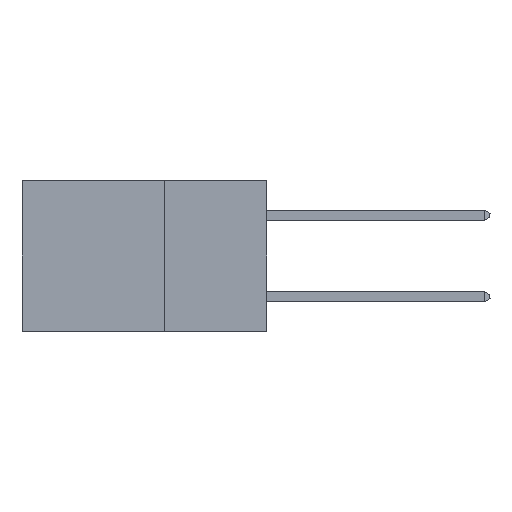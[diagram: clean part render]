
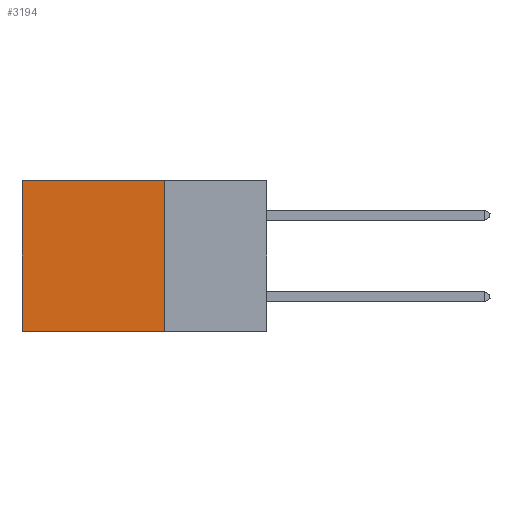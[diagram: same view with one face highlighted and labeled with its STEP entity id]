
A CAD part, left-side view. The second image highlights one B-rep face of the part: STEP entity #3194.
In plain terms, the highlighted planar face has unit normal (-1, 0, 0).
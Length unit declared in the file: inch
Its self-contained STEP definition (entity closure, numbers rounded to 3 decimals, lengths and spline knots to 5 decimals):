
#4 = ORIENTED_EDGE ( 'NONE', *, *, #1946, .F. ) ;
#265 = CARTESIAN_POINT ( 'NONE',  ( 0.2875, 0.6, 0. ) ) ;
#291 = PLANE ( 'NONE',  #7853 ) ;
#560 = CARTESIAN_POINT ( 'NONE',  ( 0.2875, 0.6, -0.37 ) ) ;
#1156 = EDGE_CURVE ( 'NONE', #4462, #20566, #4617, .T. ) ;
#1946 = EDGE_CURVE ( 'NONE', #16893, #4462, #17505, .T. ) ;
#2286 = EDGE_CURVE ( 'NONE', #20542, #20566, #9073, .T. ) ;
#2630 = LINE ( 'NONE', #16672, #20122 ) ;
#2708 = CARTESIAN_POINT ( 'NONE',  ( 0.2875, 0.25, -0.37 ) ) ;
#2721 = CARTESIAN_POINT ( 'NONE',  ( 0.2875, 0.25, 0. ) ) ;
#3194 = ADVANCED_FACE ( 'NONE', ( #3804 ), #291, .F. ) ;
#3804 = FACE_OUTER_BOUND ( 'NONE', #18959, .T. ) ;
#4462 = VERTEX_POINT ( 'NONE', #12052 ) ;
#4510 = DIRECTION ( 'NONE',  ( 0., 1., 0. ) ) ;
#4617 = LINE ( 'NONE', #2708, #19603 ) ;
#5683 = DIRECTION ( 'NONE',  ( 0., 0., -1. ) ) ;
#6805 = ORIENTED_EDGE ( 'NONE', *, *, #2286, .T. ) ;
#6942 = ORIENTED_EDGE ( 'NONE', *, *, #1156, .F. ) ;
#7347 = CARTESIAN_POINT ( 'NONE',  ( 0.2875, 0.6, 0. ) ) ;
#7853 = AXIS2_PLACEMENT_3D ( 'NONE', #10701, #19530, #16026 ) ;
#8892 = CARTESIAN_POINT ( 'NONE',  ( 0.2875, 0.25, 0. ) ) ;
#9073 = LINE ( 'NONE', #265, #14665 ) ;
#10701 = CARTESIAN_POINT ( 'NONE',  ( 0.2875, 0.25, 0. ) ) ;
#12052 = CARTESIAN_POINT ( 'NONE',  ( 0.2875, 0.25, -0.37 ) ) ;
#14665 = VECTOR ( 'NONE', #5683, 39.37008 ) ;
#15797 = DIRECTION ( 'NONE',  ( 0., 0., -1. ) ) ;
#16026 = DIRECTION ( 'NONE',  ( 0., 0., -1. ) ) ;
#16672 = CARTESIAN_POINT ( 'NONE',  ( 0.2875, 0.25, 0. ) ) ;
#16893 = VERTEX_POINT ( 'NONE', #2721 ) ;
#17505 = LINE ( 'NONE', #8892, #17576 ) ;
#17576 = VECTOR ( 'NONE', #15797, 39.37008 ) ;
#18283 = EDGE_CURVE ( 'NONE', #16893, #20542, #2630, .T. ) ;
#18959 = EDGE_LOOP ( 'NONE', ( #6805, #6942, #4, #19830 ) ) ;
#19530 = DIRECTION ( 'NONE',  ( 1., 0., 0. ) ) ;
#19603 = VECTOR ( 'NONE', #4510, 39.37008 ) ;
#19830 = ORIENTED_EDGE ( 'NONE', *, *, #18283, .T. ) ;
#19950 = DIRECTION ( 'NONE',  ( 0., 1., 0. ) ) ;
#20122 = VECTOR ( 'NONE', #19950, 39.37008 ) ;
#20542 = VERTEX_POINT ( 'NONE', #7347 ) ;
#20566 = VERTEX_POINT ( 'NONE', #560 ) ;
